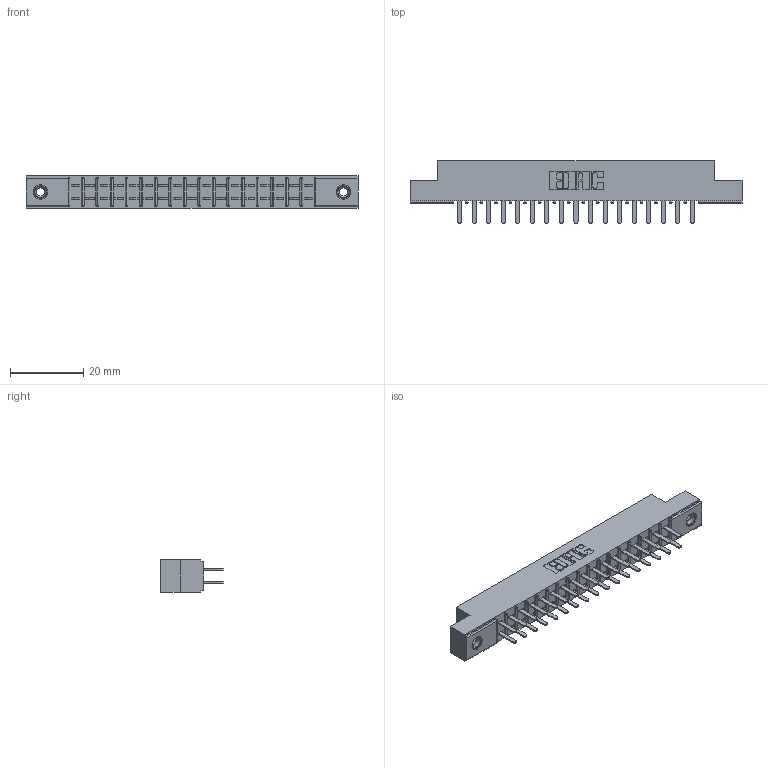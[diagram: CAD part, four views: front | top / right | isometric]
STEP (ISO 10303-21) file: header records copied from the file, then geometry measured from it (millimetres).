
FILE_DESCRIPTION (( 'STEP AP203' ), '1' );
FILE_NAME ('315-034-520-208.STEP', '2019-09-10T15:52:37', ( '' ), ( '' ), 'SwSTEP 2.0', 'SolidWorks 2016', '' );
FILE_SCHEMA (( 'CONFIG_CONTROL_DESIGN' ));
Length unit declared in the file: inch
Products named in the file (4): 315-034-520-208; 345-250-001_345-250-003-102; 305 Part_.156 Dia; 305-290-001_520
Assembly tree (37 placements, depth 2):
  315-034-520-208
    305 Part_.156 Dia
    305-290-001_520  x34
    345-250-001_345-250-003-102  x2
Bounding box: 90.37 x 17.09 x 8.71 mm (x, y, z)
Volume: 5670.2 mm3; surface area: 10451 mm2
Topology: 37 solids, 37 shells, 1740 faces, 4923 edges, 3182 vertices
Faces by surface type: plane 1018, cylinder 638, sphere 68, cone 12, torus 4
Entity records: 22515 total; most frequent: CARTESIAN_POINT 3708, ORIENTED_EDGE 3670, DIRECTION 3617, EDGE_CURVE 1835, VECTOR 1455, LINE 1455, VERTEX_POINT 1172, AXIS2_PLACEMENT_3D 1081
